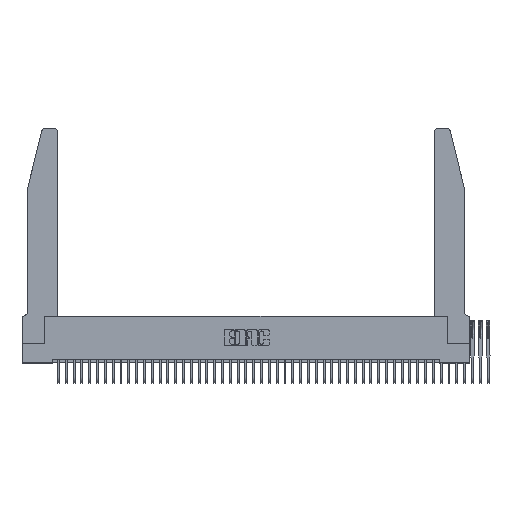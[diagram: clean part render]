
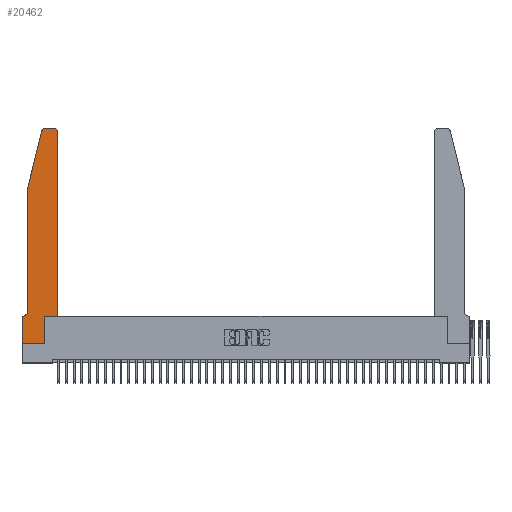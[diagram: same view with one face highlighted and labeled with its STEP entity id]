
A CAD part, top view. The second image highlights one B-rep face of the part: STEP entity #20462.
In plain terms, the highlighted planar face has unit normal (0, 0, 1).
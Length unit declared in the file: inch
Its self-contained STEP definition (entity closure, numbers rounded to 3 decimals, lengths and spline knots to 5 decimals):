
#101 = EDGE_CURVE ( 'NONE', #16708, #301, #11327, .T. ) ;
#301 = VERTEX_POINT ( 'NONE', #34913 ) ;
#535 = VECTOR ( 'NONE', #26235, 39.37008 ) ;
#773 = EDGE_CURVE ( 'NONE', #15230, #28287, #23691, .T. ) ;
#1129 = VERTEX_POINT ( 'NONE', #38939 ) ;
#1861 = ORIENTED_EDGE ( 'NONE', *, *, #15577, .T. ) ;
#1880 = CARTESIAN_POINT ( 'NONE',  ( 0.4505, 0.35, 0.37 ) ) ;
#2712 = ORIENTED_EDGE ( 'NONE', *, *, #19830, .T. ) ;
#2838 = EDGE_LOOP ( 'NONE', ( #10724, #17008, #13588, #29874, #1861, #17847, #17619, #30606, #40516, #11472, #27188, #2712 ) ) ;
#4337 = VERTEX_POINT ( 'NONE', #36837 ) ;
#5111 = DIRECTION ( 'NONE',  ( 1., 0., 0. ) ) ;
#5565 = EDGE_CURVE ( 'NONE', #18441, #33857, #40376, .T. ) ;
#5794 = VECTOR ( 'NONE', #13899, 39.37008 ) ;
#6071 = EDGE_CURVE ( 'NONE', #32689, #16708, #29133, .T. ) ;
#7156 = CARTESIAN_POINT ( 'NONE',  ( 0.2865, 0.35, 0.37 ) ) ;
#8379 = DIRECTION ( 'NONE',  ( 0., 0., -1. ) ) ;
#8685 = CARTESIAN_POINT ( 'NONE',  ( 0.0755, 2., 0.37 ) ) ;
#10688 = CARTESIAN_POINT ( 'NONE',  ( 0.4505, 0.35, 0.37 ) ) ;
#10724 = ORIENTED_EDGE ( 'NONE', *, *, #5565, .T. ) ;
#10905 = LINE ( 'NONE', #13324, #35068 ) ;
#11241 = CIRCLE ( 'NONE', #31502, 0.03 ) ;
#11258 = CARTESIAN_POINT ( 'NONE',  ( 0., 0.35, 0.37 ) ) ;
#11327 = LINE ( 'NONE', #8685, #18808 ) ;
#11330 = CARTESIAN_POINT ( 'NONE',  ( 0.0755, 2., 0.37 ) ) ;
#11472 = ORIENTED_EDGE ( 'NONE', *, *, #40479, .T. ) ;
#11646 = DIRECTION ( 'NONE',  ( 0., 0., 1. ) ) ;
#12768 = VECTOR ( 'NONE', #5111, 39.37008 ) ;
#13324 = CARTESIAN_POINT ( 'NONE',  ( 0., 0., 0.37 ) ) ;
#13436 = EDGE_CURVE ( 'NONE', #33857, #32689, #23434, .T. ) ;
#13588 = ORIENTED_EDGE ( 'NONE', *, *, #6071, .T. ) ;
#13899 = DIRECTION ( 'NONE',  ( 0., 1., 0. ) ) ;
#14272 = DIRECTION ( 'NONE',  ( 0., 0., 1. ) ) ;
#14987 = DIRECTION ( 'NONE',  ( 0., -1., 0. ) ) ;
#15230 = VERTEX_POINT ( 'NONE', #22508 ) ;
#15245 = VECTOR ( 'NONE', #18566, 39.37008 ) ;
#15577 = EDGE_CURVE ( 'NONE', #301, #15230, #35460, .T. ) ;
#15580 = VERTEX_POINT ( 'NONE', #17875 ) ;
#16301 = VECTOR ( 'NONE', #30852, 39.37008 ) ;
#16708 = VERTEX_POINT ( 'NONE', #11330 ) ;
#16715 = CARTESIAN_POINT ( 'NONE',  ( 0.25487, 2.72718, 0.37 ) ) ;
#17008 = ORIENTED_EDGE ( 'NONE', *, *, #13436, .T. ) ;
#17619 = ORIENTED_EDGE ( 'NONE', *, *, #23234, .T. ) ;
#17792 = EDGE_CURVE ( 'NONE', #27237, #1129, #10905, .T. ) ;
#17847 = ORIENTED_EDGE ( 'NONE', *, *, #773, .T. ) ;
#17875 = CARTESIAN_POINT ( 'NONE',  ( 0.2865, 0.35, 0.37 ) ) ;
#17944 = CARTESIAN_POINT ( 'NONE',  ( 0.4205, 2.72, 0.37 ) ) ;
#18441 = VERTEX_POINT ( 'NONE', #23579 ) ;
#18566 = DIRECTION ( 'NONE',  ( -1., 0., 0. ) ) ;
#18808 = VECTOR ( 'NONE', #14987, 39.37008 ) ;
#19830 = EDGE_CURVE ( 'NONE', #4337, #18441, #11241, .T. ) ;
#20260 = DIRECTION ( 'NONE',  ( 0., -1., 0. ) ) ;
#20462 = ADVANCED_FACE ( 'NONE', ( #34844 ), #27442, .T. ) ;
#21187 = DIRECTION ( 'NONE',  ( 1., 0., 0. ) ) ;
#21403 = VECTOR ( 'NONE', #20260, 39.37008 ) ;
#21912 = EDGE_CURVE ( 'NONE', #1129, #15580, #33363, .T. ) ;
#22508 = CARTESIAN_POINT ( 'NONE',  ( 0.0055, 0.35, 0.37 ) ) ;
#23234 = EDGE_CURVE ( 'NONE', #28287, #27237, #29718, .T. ) ;
#23434 = CIRCLE ( 'NONE', #29536, 0.03 ) ;
#23579 = CARTESIAN_POINT ( 'NONE',  ( 0.4205, 2.75, 0.37 ) ) ;
#23691 = LINE ( 'NONE', #31090, #15245 ) ;
#23779 = LINE ( 'NONE', #10688, #5794 ) ;
#23820 = DIRECTION ( 'NONE',  ( -0.239, -0.971, 0. ) ) ;
#23869 = EDGE_CURVE ( 'NONE', #32553, #4337, #23779, .T. ) ;
#24565 = CARTESIAN_POINT ( 'NONE',  ( 0.2605, 2.75, 0.37 ) ) ;
#26235 = DIRECTION ( 'NONE',  ( 0., 1., 0. ) ) ;
#27188 = ORIENTED_EDGE ( 'NONE', *, *, #23869, .T. ) ;
#27237 = VERTEX_POINT ( 'NONE', #33525 ) ;
#27426 = CARTESIAN_POINT ( 'NONE',  ( 0.0055, 0.42, 0.37 ) ) ;
#27442 = PLANE ( 'NONE',  #36205 ) ;
#28287 = VERTEX_POINT ( 'NONE', #11258 ) ;
#29133 = LINE ( 'NONE', #36247, #36450 ) ;
#29536 = AXIS2_PLACEMENT_3D ( 'NONE', #33177, #14272, #36294 ) ;
#29712 = CARTESIAN_POINT ( 'NONE',  ( 0., 0., 0.37 ) ) ;
#29718 = LINE ( 'NONE', #29712, #21403 ) ;
#29874 = ORIENTED_EDGE ( 'NONE', *, *, #101, .T. ) ;
#30563 = DIRECTION ( 'NONE',  ( -1., 0., 0. ) ) ;
#30606 = ORIENTED_EDGE ( 'NONE', *, *, #17792, .T. ) ;
#30852 = DIRECTION ( 'NONE',  ( -1., 0., 0. ) ) ;
#31090 = CARTESIAN_POINT ( 'NONE',  ( 0.0755, 0.35, 0.37 ) ) ;
#31502 = AXIS2_PLACEMENT_3D ( 'NONE', #17944, #39863, #21187 ) ;
#31752 = CARTESIAN_POINT ( 'NONE',  ( 0.4505, 0.35, 0.37 ) ) ;
#32198 = CARTESIAN_POINT ( 'NONE',  ( 0.284, 2.75, 0.37 ) ) ;
#32553 = VERTEX_POINT ( 'NONE', #31752 ) ;
#32689 = VERTEX_POINT ( 'NONE', #16715 ) ;
#33177 = CARTESIAN_POINT ( 'NONE',  ( 0.284, 2.72, 0.37 ) ) ;
#33363 = LINE ( 'NONE', #7156, #535 ) ;
#33525 = CARTESIAN_POINT ( 'NONE',  ( 0., 0., 0.37 ) ) ;
#33716 = DIRECTION ( 'NONE',  ( 1., 0., 0. ) ) ;
#33857 = VERTEX_POINT ( 'NONE', #32198 ) ;
#34844 = FACE_OUTER_BOUND ( 'NONE', #2838, .T. ) ;
#34913 = CARTESIAN_POINT ( 'NONE',  ( 0.0755, 0.42, 0.37 ) ) ;
#35068 = VECTOR ( 'NONE', #38496, 39.37008 ) ;
#35312 = AXIS2_PLACEMENT_3D ( 'NONE', #27426, #8379, #30563 ) ;
#35460 = CIRCLE ( 'NONE', #35312, 0.07 ) ;
#36205 = AXIS2_PLACEMENT_3D ( 'NONE', #39814, #11646, #33716 ) ;
#36247 = CARTESIAN_POINT ( 'NONE',  ( 0.0755, 2., 0.37 ) ) ;
#36294 = DIRECTION ( 'NONE',  ( 1., 0., 0. ) ) ;
#36450 = VECTOR ( 'NONE', #23820, 39.37008 ) ;
#36837 = CARTESIAN_POINT ( 'NONE',  ( 0.4505, 2.72, 0.37 ) ) ;
#37886 = LINE ( 'NONE', #1880, #12768 ) ;
#38496 = DIRECTION ( 'NONE',  ( 1., 0., 0. ) ) ;
#38939 = CARTESIAN_POINT ( 'NONE',  ( 0.2865, 0., 0.37 ) ) ;
#39814 = CARTESIAN_POINT ( 'NONE',  ( 0., 0.35, 0.37 ) ) ;
#39863 = DIRECTION ( 'NONE',  ( 0., 0., 1. ) ) ;
#40376 = LINE ( 'NONE', #24565, #16301 ) ;
#40479 = EDGE_CURVE ( 'NONE', #15580, #32553, #37886, .T. ) ;
#40516 = ORIENTED_EDGE ( 'NONE', *, *, #21912, .T. ) ;
